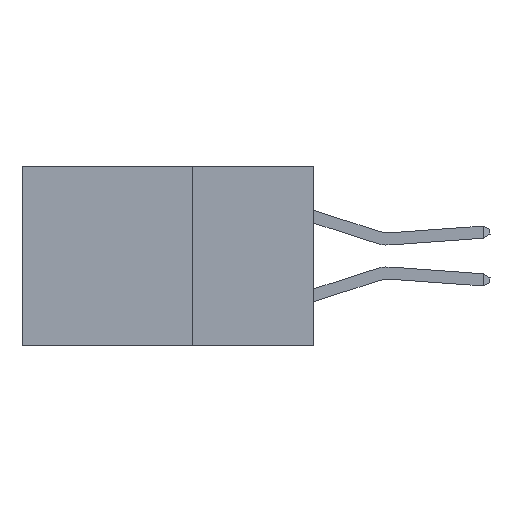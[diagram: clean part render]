
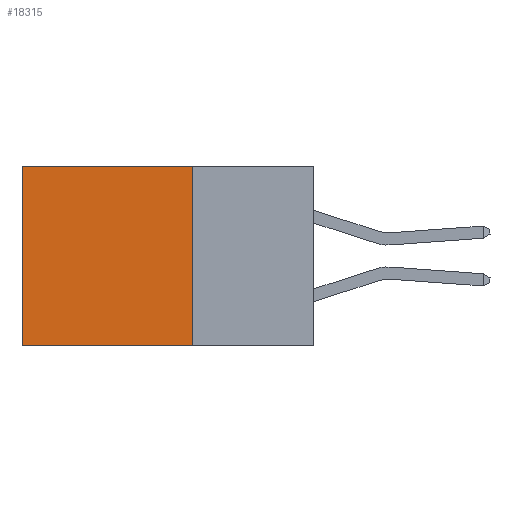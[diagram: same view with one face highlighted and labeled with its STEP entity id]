
A CAD part, left-side view. The second image highlights one B-rep face of the part: STEP entity #18315.
In plain terms, the highlighted planar face has unit normal (-1, 0, 0).
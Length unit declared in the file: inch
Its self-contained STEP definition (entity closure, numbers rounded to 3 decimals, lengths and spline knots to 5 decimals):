
#64 = ORIENTED_EDGE ( 'NONE', *, *, #11022, .F. ) ;
#1873 = DIRECTION ( 'NONE',  ( 0., 0., -1. ) ) ;
#4543 = CARTESIAN_POINT ( 'NONE',  ( 0.2875, 0.6, 0. ) ) ;
#5223 = DIRECTION ( 'NONE',  ( 0., 0., -1. ) ) ;
#5746 = DIRECTION ( 'NONE',  ( 0., 1., 0. ) ) ;
#5747 = CARTESIAN_POINT ( 'NONE',  ( 0.2875, 0.6, 0. ) ) ;
#6622 = EDGE_CURVE ( 'NONE', #15697, #19735, #27264, .T. ) ;
#8402 = VERTEX_POINT ( 'NONE', #5747 ) ;
#9304 = DIRECTION ( 'NONE',  ( 1., 0., 0. ) ) ;
#11022 = EDGE_CURVE ( 'NONE', #19735, #14260, #29665, .T. ) ;
#12306 = DIRECTION ( 'NONE',  ( 0., 0., -1. ) ) ;
#12465 = EDGE_CURVE ( 'NONE', #15697, #8402, #29134, .T. ) ;
#14260 = VERTEX_POINT ( 'NONE', #23996 ) ;
#14420 = DIRECTION ( 'NONE',  ( 0., 1., 0. ) ) ;
#14473 = PLANE ( 'NONE',  #24755 ) ;
#14747 = EDGE_CURVE ( 'NONE', #8402, #14260, #19105, .T. ) ;
#15437 = CARTESIAN_POINT ( 'NONE',  ( 0.2875, 0.25, -0.37 ) ) ;
#15697 = VERTEX_POINT ( 'NONE', #16208 ) ;
#16208 = CARTESIAN_POINT ( 'NONE',  ( 0.2875, 0.25, 0. ) ) ;
#18315 = ADVANCED_FACE ( 'NONE', ( #19271 ), #14473, .F. ) ;
#19105 = LINE ( 'NONE', #4543, #31078 ) ;
#19271 = FACE_OUTER_BOUND ( 'NONE', #23000, .T. ) ;
#19735 = VERTEX_POINT ( 'NONE', #15437 ) ;
#20044 = CARTESIAN_POINT ( 'NONE',  ( 0.2875, 0.25, 0. ) ) ;
#21410 = ORIENTED_EDGE ( 'NONE', *, *, #12465, .T. ) ;
#21805 = CARTESIAN_POINT ( 'NONE',  ( 0.2875, 0.25, 0. ) ) ;
#23000 = EDGE_LOOP ( 'NONE', ( #34079, #64, #31931, #21410 ) ) ;
#23341 = VECTOR ( 'NONE', #5746, 39.37008 ) ;
#23996 = CARTESIAN_POINT ( 'NONE',  ( 0.2875, 0.6, -0.37 ) ) ;
#24291 = VECTOR ( 'NONE', #14420, 39.37008 ) ;
#24755 = AXIS2_PLACEMENT_3D ( 'NONE', #20044, #9304, #12306 ) ;
#26013 = CARTESIAN_POINT ( 'NONE',  ( 0.2875, 0.25, 0. ) ) ;
#27264 = LINE ( 'NONE', #26013, #31820 ) ;
#29134 = LINE ( 'NONE', #21805, #23341 ) ;
#29665 = LINE ( 'NONE', #29908, #24291 ) ;
#29908 = CARTESIAN_POINT ( 'NONE',  ( 0.2875, 0.25, -0.37 ) ) ;
#31078 = VECTOR ( 'NONE', #1873, 39.37008 ) ;
#31820 = VECTOR ( 'NONE', #5223, 39.37008 ) ;
#31931 = ORIENTED_EDGE ( 'NONE', *, *, #6622, .F. ) ;
#34079 = ORIENTED_EDGE ( 'NONE', *, *, #14747, .T. ) ;
